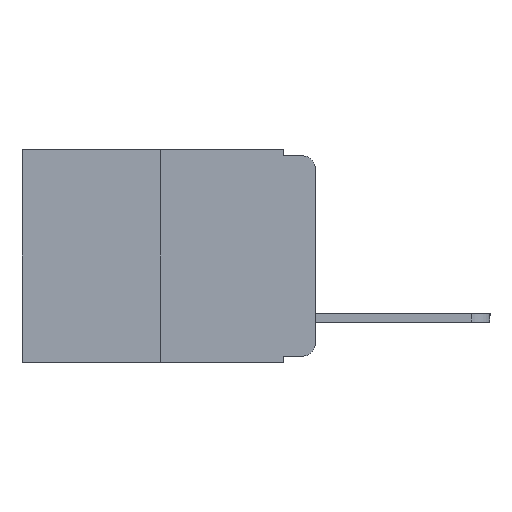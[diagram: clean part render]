
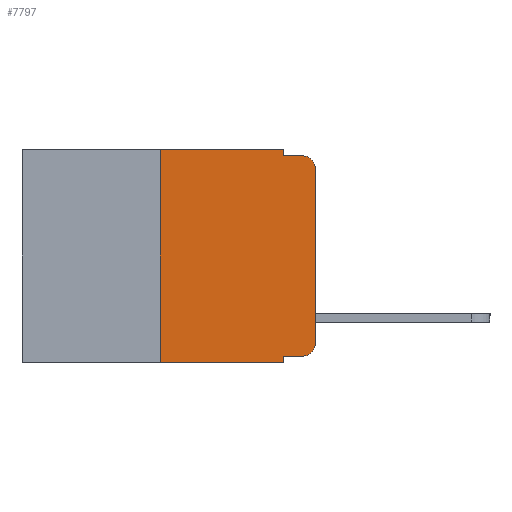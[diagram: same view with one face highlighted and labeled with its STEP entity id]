
A CAD part, left-side view. The second image highlights one B-rep face of the part: STEP entity #7797.
In plain terms, the highlighted planar face has unit normal (-1, 0, 0).
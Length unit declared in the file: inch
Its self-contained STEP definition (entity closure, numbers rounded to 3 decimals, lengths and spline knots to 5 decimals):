
#233 = FACE_OUTER_BOUND ( 'NONE', #20577, .T. ) ;
#288 = DIRECTION ( 'NONE',  ( 0., 0., 1. ) ) ;
#445 = VERTEX_POINT ( 'NONE', #12354 ) ;
#528 = ORIENTED_EDGE ( 'NONE', *, *, #24532, .T. ) ;
#531 = CARTESIAN_POINT ( 'NONE',  ( 0., 0., 0. ) ) ;
#663 = DIRECTION ( 'NONE',  ( 0., -1., 0. ) ) ;
#739 = ORIENTED_EDGE ( 'NONE', *, *, #23239, .T. ) ;
#749 = CIRCLE ( 'NONE', #5077, 0.02 ) ;
#1424 = ORIENTED_EDGE ( 'NONE', *, *, #21917, .F. ) ;
#1480 = CARTESIAN_POINT ( 'NONE',  ( 0., 0.473, 0. ) ) ;
#1769 = VERTEX_POINT ( 'NONE', #18856 ) ;
#2925 = AXIS2_PLACEMENT_3D ( 'NONE', #1480, #15605, #3630 ) ;
#3104 = VECTOR ( 'NONE', #16695, 39.37008 ) ;
#3164 = DIRECTION ( 'NONE',  ( 0., 0., -1. ) ) ;
#3259 = CARTESIAN_POINT ( 'NONE',  ( 0., 0.473, -0.343 ) ) ;
#3630 = DIRECTION ( 'NONE',  ( 0., 0., -1. ) ) ;
#3668 = VECTOR ( 'NONE', #663, 39.37008 ) ;
#4027 = VECTOR ( 'NONE', #8716, 39.37008 ) ;
#4166 = CARTESIAN_POINT ( 'NONE',  ( 0., 0.051, 0. ) ) ;
#4247 = DIRECTION ( 'NONE',  ( -1., 0., 0. ) ) ;
#4249 = DIRECTION ( 'NONE',  ( 0., 0., -1. ) ) ;
#4781 = DIRECTION ( 'NONE',  ( 0., -1., 0. ) ) ;
#5077 = AXIS2_PLACEMENT_3D ( 'NONE', #16197, #4247, #18188 ) ;
#5292 = CARTESIAN_POINT ( 'NONE',  ( 0., 0.25, 0. ) ) ;
#5441 = VERTEX_POINT ( 'NONE', #11914 ) ;
#5463 = ORIENTED_EDGE ( 'NONE', *, *, #19336, .F. ) ;
#5550 = CIRCLE ( 'NONE', #6008, 0.02 ) ;
#5800 = LINE ( 'NONE', #4166, #20387 ) ;
#6008 = AXIS2_PLACEMENT_3D ( 'NONE', #19197, #7304, #21149 ) ;
#6392 = CARTESIAN_POINT ( 'NONE',  ( 0., 0.051, -0.01 ) ) ;
#6405 = ORIENTED_EDGE ( 'NONE', *, *, #13329, .F. ) ;
#6733 = CARTESIAN_POINT ( 'NONE',  ( 0., 0.051, -0.343 ) ) ;
#7304 = DIRECTION ( 'NONE',  ( -1., 0., 0. ) ) ;
#7695 = EDGE_CURVE ( 'NONE', #13762, #12079, #8326, .T. ) ;
#7797 = ADVANCED_FACE ( 'NONE', ( #233 ), #11613, .F. ) ;
#8326 = LINE ( 'NONE', #3259, #13579 ) ;
#8716 = DIRECTION ( 'NONE',  ( 0., -1., 0. ) ) ;
#9032 = LINE ( 'NONE', #10853, #3668 ) ;
#9138 = VERTEX_POINT ( 'NONE', #9981 ) ;
#9384 = LINE ( 'NONE', #12605, #4027 ) ;
#9981 = CARTESIAN_POINT ( 'NONE',  ( 0., 0.02, -0.01 ) ) ;
#10853 = CARTESIAN_POINT ( 'NONE',  ( 0., 0.473, 0. ) ) ;
#11348 = EDGE_CURVE ( 'NONE', #445, #1769, #749, .T. ) ;
#11613 = PLANE ( 'NONE',  #2925 ) ;
#11914 = CARTESIAN_POINT ( 'NONE',  ( 0., 0.051, 0. ) ) ;
#12079 = VERTEX_POINT ( 'NONE', #6733 ) ;
#12354 = CARTESIAN_POINT ( 'NONE',  ( 0., 0.02, -0.333 ) ) ;
#12605 = CARTESIAN_POINT ( 'NONE',  ( 0., 0.051, -0.333 ) ) ;
#12646 = EDGE_CURVE ( 'NONE', #19400, #445, #9384, .T. ) ;
#13329 = EDGE_CURVE ( 'NONE', #14696, #5441, #9032, .T. ) ;
#13579 = VECTOR ( 'NONE', #19267, 39.37008 ) ;
#13762 = VERTEX_POINT ( 'NONE', #14273 ) ;
#13863 = VECTOR ( 'NONE', #3164, 39.37008 ) ;
#14273 = CARTESIAN_POINT ( 'NONE',  ( 0., 0.25, -0.343 ) ) ;
#14696 = VERTEX_POINT ( 'NONE', #5292 ) ;
#14712 = CARTESIAN_POINT ( 'NONE',  ( 0., 0.051, -0.01 ) ) ;
#14800 = ORIENTED_EDGE ( 'NONE', *, *, #17968, .F. ) ;
#14966 = ORIENTED_EDGE ( 'NONE', *, *, #15313, .F. ) ;
#15313 = EDGE_CURVE ( 'NONE', #19400, #12079, #23744, .T. ) ;
#15605 = DIRECTION ( 'NONE',  ( 1., 0., 0. ) ) ;
#15744 = ORIENTED_EDGE ( 'NONE', *, *, #7695, .T. ) ;
#16041 = LINE ( 'NONE', #22322, #21294 ) ;
#16197 = CARTESIAN_POINT ( 'NONE',  ( 0., 0.02, -0.313 ) ) ;
#16695 = DIRECTION ( 'NONE',  ( 0., 0., 1. ) ) ;
#17395 = ORIENTED_EDGE ( 'NONE', *, *, #11348, .T. ) ;
#17408 = LINE ( 'NONE', #14712, #21422 ) ;
#17733 = VERTEX_POINT ( 'NONE', #21571 ) ;
#17968 = EDGE_CURVE ( 'NONE', #13762, #14696, #16041, .T. ) ;
#18188 = DIRECTION ( 'NONE',  ( 0., 0., -1. ) ) ;
#18856 = CARTESIAN_POINT ( 'NONE',  ( 0., 0., -0.313 ) ) ;
#19197 = CARTESIAN_POINT ( 'NONE',  ( 0., 0.02, -0.03 ) ) ;
#19267 = DIRECTION ( 'NONE',  ( 0., -1., 0. ) ) ;
#19336 = EDGE_CURVE ( 'NONE', #5441, #19956, #5800, .T. ) ;
#19400 = VERTEX_POINT ( 'NONE', #20372 ) ;
#19705 = LINE ( 'NONE', #531, #3104 ) ;
#19956 = VERTEX_POINT ( 'NONE', #6392 ) ;
#20372 = CARTESIAN_POINT ( 'NONE',  ( 0., 0.051, -0.333 ) ) ;
#20387 = VECTOR ( 'NONE', #4249, 39.37008 ) ;
#20577 = EDGE_LOOP ( 'NONE', ( #528, #739, #1424, #5463, #6405, #14800, #15744, #14966, #24947, #17395 ) ) ;
#21149 = DIRECTION ( 'NONE',  ( 0., 0., -1. ) ) ;
#21294 = VECTOR ( 'NONE', #288, 39.37008 ) ;
#21422 = VECTOR ( 'NONE', #4781, 39.37008 ) ;
#21571 = CARTESIAN_POINT ( 'NONE',  ( 0., 0., -0.03 ) ) ;
#21917 = EDGE_CURVE ( 'NONE', #19956, #9138, #17408, .T. ) ;
#22322 = CARTESIAN_POINT ( 'NONE',  ( 0., 0.25, 0. ) ) ;
#23077 = CARTESIAN_POINT ( 'NONE',  ( 0., 0.051, 0. ) ) ;
#23239 = EDGE_CURVE ( 'NONE', #17733, #9138, #5550, .T. ) ;
#23744 = LINE ( 'NONE', #23077, #13863 ) ;
#24532 = EDGE_CURVE ( 'NONE', #1769, #17733, #19705, .T. ) ;
#24947 = ORIENTED_EDGE ( 'NONE', *, *, #12646, .T. ) ;
